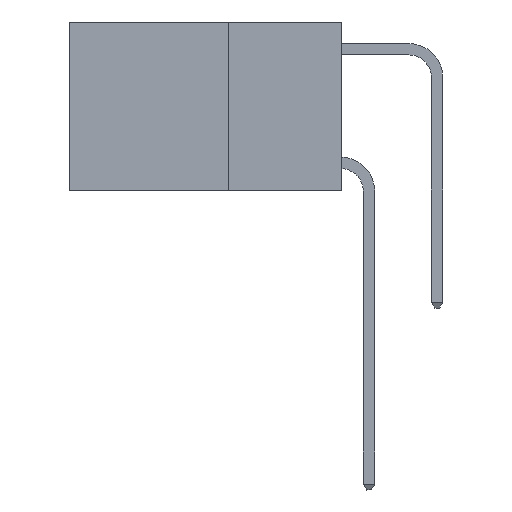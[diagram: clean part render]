
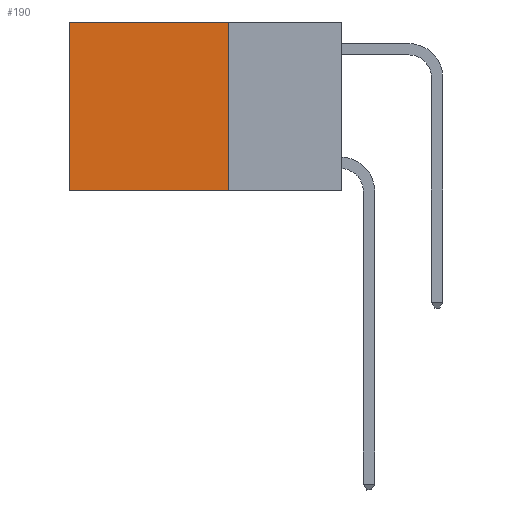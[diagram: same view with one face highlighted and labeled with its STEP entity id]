
A CAD part, left-side view. The second image highlights one B-rep face of the part: STEP entity #190.
In plain terms, the highlighted planar face has unit normal (-1, 0, 0).
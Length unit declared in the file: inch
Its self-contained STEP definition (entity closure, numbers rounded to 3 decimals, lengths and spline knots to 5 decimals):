
#25 = VECTOR ( 'NONE', #1436, 39.37008 ) ;
#118 = ORIENTED_EDGE ( 'NONE', *, *, #12523, .T. ) ;
#190 = ADVANCED_FACE ( 'NONE', ( #10961 ), #16707, .F. ) ;
#689 = AXIS2_PLACEMENT_3D ( 'NONE', #9435, #3614, #3706 ) ;
#1179 = EDGE_LOOP ( 'NONE', ( #118, #12402, #2302, #18343 ) ) ;
#1190 = LINE ( 'NONE', #3766, #15347 ) ;
#1436 = DIRECTION ( 'NONE',  ( 0., 0., -1. ) ) ;
#2302 = ORIENTED_EDGE ( 'NONE', *, *, #15799, .F. ) ;
#2604 = VECTOR ( 'NONE', #8945, 39.37008 ) ;
#3614 = DIRECTION ( 'NONE',  ( 1., 0., 0. ) ) ;
#3706 = DIRECTION ( 'NONE',  ( 0., 0., -1. ) ) ;
#3766 = CARTESIAN_POINT ( 'NONE',  ( 0.2625, 0.25, 0. ) ) ;
#3811 = CARTESIAN_POINT ( 'NONE',  ( 0.2625, 0.25, 0. ) ) ;
#4603 = VERTEX_POINT ( 'NONE', #18043 ) ;
#8344 = DIRECTION ( 'NONE',  ( 0., 1., 0. ) ) ;
#8651 = VECTOR ( 'NONE', #16603, 39.37008 ) ;
#8945 = DIRECTION ( 'NONE',  ( 0., 1., 0. ) ) ;
#9435 = CARTESIAN_POINT ( 'NONE',  ( 0.2625, 0.25, 0. ) ) ;
#10402 = LINE ( 'NONE', #10587, #25 ) ;
#10587 = CARTESIAN_POINT ( 'NONE',  ( 0.2625, 0.6, 0. ) ) ;
#10762 = CARTESIAN_POINT ( 'NONE',  ( 0.2625, 0.25, 0. ) ) ;
#10961 = FACE_OUTER_BOUND ( 'NONE', #1179, .T. ) ;
#11407 = VERTEX_POINT ( 'NONE', #18125 ) ;
#12402 = ORIENTED_EDGE ( 'NONE', *, *, #17717, .F. ) ;
#12523 = EDGE_CURVE ( 'NONE', #4603, #11407, #10402, .T. ) ;
#12569 = CARTESIAN_POINT ( 'NONE',  ( 0.2625, 0.25, -0.37 ) ) ;
#13719 = LINE ( 'NONE', #18103, #2604 ) ;
#13813 = VERTEX_POINT ( 'NONE', #3811 ) ;
#14916 = EDGE_CURVE ( 'NONE', #13813, #4603, #1190, .T. ) ;
#15347 = VECTOR ( 'NONE', #8344, 39.37008 ) ;
#15799 = EDGE_CURVE ( 'NONE', #13813, #15831, #18022, .T. ) ;
#15831 = VERTEX_POINT ( 'NONE', #12569 ) ;
#16603 = DIRECTION ( 'NONE',  ( 0., 0., -1. ) ) ;
#16707 = PLANE ( 'NONE',  #689 ) ;
#17717 = EDGE_CURVE ( 'NONE', #15831, #11407, #13719, .T. ) ;
#18022 = LINE ( 'NONE', #10762, #8651 ) ;
#18043 = CARTESIAN_POINT ( 'NONE',  ( 0.2625, 0.6, 0. ) ) ;
#18103 = CARTESIAN_POINT ( 'NONE',  ( 0.2625, 0.25, -0.37 ) ) ;
#18125 = CARTESIAN_POINT ( 'NONE',  ( 0.2625, 0.6, -0.37 ) ) ;
#18343 = ORIENTED_EDGE ( 'NONE', *, *, #14916, .T. ) ;
